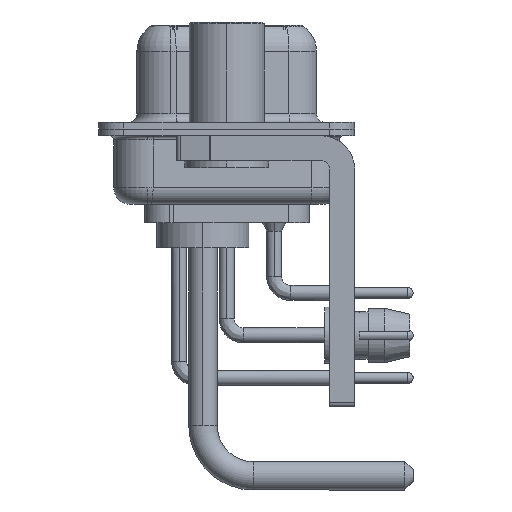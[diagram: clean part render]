
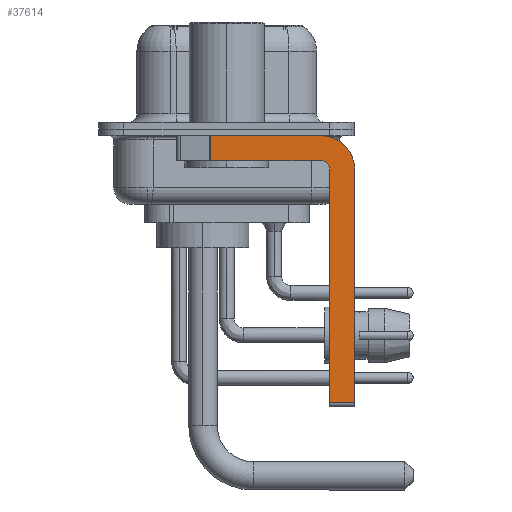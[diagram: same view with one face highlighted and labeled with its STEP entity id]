
A CAD part, left-side view. The second image highlights one B-rep face of the part: STEP entity #37614.
In plain terms, the highlighted planar face has unit normal (-1, 0, 0).
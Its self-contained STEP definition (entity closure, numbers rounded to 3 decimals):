
#546 = CARTESIAN_POINT ( 'NONE',  ( -2.9, -5.65, -1.9 ) ) ;
#789 = DIRECTION ( 'NONE',  ( 1., 0., 0. ) ) ;
#1127 = VERTEX_POINT ( 'NONE', #13484 ) ;
#1610 = CIRCLE ( 'NONE', #26227, 0.5 ) ;
#2051 = LINE ( 'NONE', #8022, #18086 ) ;
#2965 = ORIENTED_EDGE ( 'NONE', *, *, #15737, .F. ) ;
#4346 = EDGE_CURVE ( 'NONE', #27550, #26212, #2051, .T. ) ;
#4681 = EDGE_CURVE ( 'NONE', #1127, #25246, #27823, .T. ) ;
#4868 = ORIENTED_EDGE ( 'NONE', *, *, #4346, .F. ) ;
#5138 = VERTEX_POINT ( 'NONE', #11772 ) ;
#5916 = DIRECTION ( 'NONE',  ( 0., 0., -1. ) ) ;
#6374 = CARTESIAN_POINT ( 'NONE',  ( -2.9, -7.65, -2.4 ) ) ;
#6392 = FACE_OUTER_BOUND ( 'NONE', #23488, .T. ) ;
#6536 = DIRECTION ( 'NONE',  ( 0., -1., 0. ) ) ;
#6730 = LINE ( 'NONE', #27143, #37229 ) ;
#6778 = CARTESIAN_POINT ( 'NONE',  ( -2.9, -5.65, -16.35 ) ) ;
#6958 = CARTESIAN_POINT ( 'NONE',  ( -2.9, -5.65, -0.4 ) ) ;
#8022 = CARTESIAN_POINT ( 'NONE',  ( -2.9, -7.65, -2.4 ) ) ;
#9018 = DIRECTION ( 'NONE',  ( 0., 1., 0. ) ) ;
#9296 = PLANE ( 'NONE',  #32718 ) ;
#10282 = DIRECTION ( 'NONE',  ( -1., 0., 0. ) ) ;
#10470 = DIRECTION ( 'NONE',  ( 0., 0., 1. ) ) ;
#11283 = VERTEX_POINT ( 'NONE', #15346 ) ;
#11538 = AXIS2_PLACEMENT_3D ( 'NONE', #23483, #32174, #20583 ) ;
#11772 = CARTESIAN_POINT ( 'NONE',  ( -2.9, 0.978, -0.4 ) ) ;
#12202 = CARTESIAN_POINT ( 'NONE',  ( -2.9, -5.65, -2.4 ) ) ;
#13180 = CARTESIAN_POINT ( 'NONE',  ( -2.9, -5.65, -2.4 ) ) ;
#13484 = CARTESIAN_POINT ( 'NONE',  ( -2.9, -6.15, -16.35 ) ) ;
#14615 = CIRCLE ( 'NONE', #11538, 2. ) ;
#14875 = VERTEX_POINT ( 'NONE', #546 ) ;
#15346 = CARTESIAN_POINT ( 'NONE',  ( -2.9, 0.978, -1.9 ) ) ;
#15737 = EDGE_CURVE ( 'NONE', #5138, #33607, #6730, .T. ) ;
#16356 = EDGE_CURVE ( 'NONE', #14875, #11283, #21506, .T. ) ;
#18086 = VECTOR ( 'NONE', #19953, 1000. ) ;
#18409 = DIRECTION ( 'NONE',  ( 0., 0., 1. ) ) ;
#18537 = LINE ( 'NONE', #6778, #21551 ) ;
#19953 = DIRECTION ( 'NONE',  ( 0., 0., -1. ) ) ;
#20074 = VECTOR ( 'NONE', #5916, 1000. ) ;
#20583 = DIRECTION ( 'NONE',  ( 0., 0., -1. ) ) ;
#21506 = LINE ( 'NONE', #33090, #23715 ) ;
#21551 = VECTOR ( 'NONE', #36066, 1000. ) ;
#22301 = ORIENTED_EDGE ( 'NONE', *, *, #32554, .F. ) ;
#23483 = CARTESIAN_POINT ( 'NONE',  ( -2.9, -5.65, -2.4 ) ) ;
#23488 = EDGE_LOOP ( 'NONE', ( #2965, #25134, #23808, #36417, #29941, #35959, #4868, #22301 ) ) ;
#23715 = VECTOR ( 'NONE', #9018, 1000. ) ;
#23738 = DIRECTION ( 'NONE',  ( 0., 0., -1. ) ) ;
#23808 = ORIENTED_EDGE ( 'NONE', *, *, #16356, .F. ) ;
#25134 = ORIENTED_EDGE ( 'NONE', *, *, #29920, .T. ) ;
#25246 = VERTEX_POINT ( 'NONE', #26609 ) ;
#26212 = VERTEX_POINT ( 'NONE', #35007 ) ;
#26227 = AXIS2_PLACEMENT_3D ( 'NONE', #13180, #10282, #10470 ) ;
#26609 = CARTESIAN_POINT ( 'NONE',  ( -2.9, -6.15, -2.4 ) ) ;
#27143 = CARTESIAN_POINT ( 'NONE',  ( -2.9, 3., -0.4 ) ) ;
#27229 = VECTOR ( 'NONE', #18409, 1000. ) ;
#27550 = VERTEX_POINT ( 'NONE', #6374 ) ;
#27823 = LINE ( 'NONE', #34002, #27229 ) ;
#29920 = EDGE_CURVE ( 'NONE', #5138, #11283, #32318, .T. ) ;
#29941 = ORIENTED_EDGE ( 'NONE', *, *, #4681, .F. ) ;
#31735 = EDGE_CURVE ( 'NONE', #25246, #14875, #1610, .T. ) ;
#32174 = DIRECTION ( 'NONE',  ( 1., 0., 0. ) ) ;
#32318 = LINE ( 'NONE', #35766, #20074 ) ;
#32554 = EDGE_CURVE ( 'NONE', #33607, #27550, #14615, .T. ) ;
#32718 = AXIS2_PLACEMENT_3D ( 'NONE', #12202, #789, #23738 ) ;
#33090 = CARTESIAN_POINT ( 'NONE',  ( -2.9, -5.65, -1.9 ) ) ;
#33607 = VERTEX_POINT ( 'NONE', #6958 ) ;
#34002 = CARTESIAN_POINT ( 'NONE',  ( -2.9, -6.15, -16.6 ) ) ;
#35007 = CARTESIAN_POINT ( 'NONE',  ( -2.9, -7.65, -16.35 ) ) ;
#35508 = EDGE_CURVE ( 'NONE', #1127, #26212, #18537, .T. ) ;
#35766 = CARTESIAN_POINT ( 'NONE',  ( -2.9, 0.978, -1.9 ) ) ;
#35959 = ORIENTED_EDGE ( 'NONE', *, *, #35508, .T. ) ;
#36066 = DIRECTION ( 'NONE',  ( 0., -1., 0. ) ) ;
#36417 = ORIENTED_EDGE ( 'NONE', *, *, #31735, .F. ) ;
#37229 = VECTOR ( 'NONE', #6536, 1000. ) ;
#37614 = ADVANCED_FACE ( 'NONE', ( #6392 ), #9296, .F. ) ;
